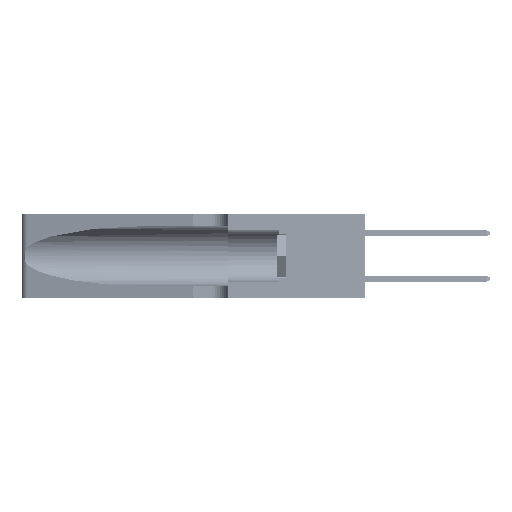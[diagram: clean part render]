
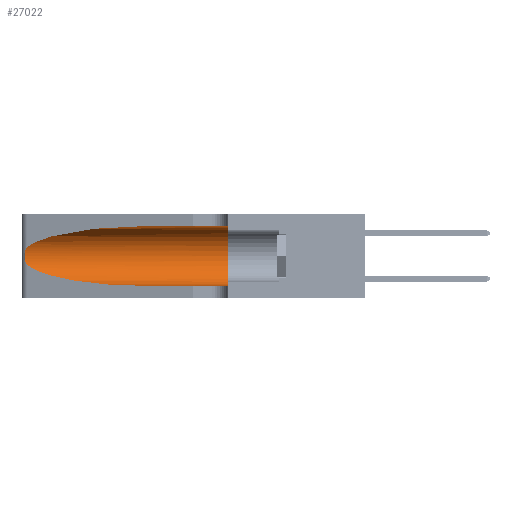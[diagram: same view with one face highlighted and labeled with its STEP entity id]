
A CAD part, left-side view. The second image highlights one B-rep face of the part: STEP entity #27022.
In plain terms, the highlighted cylindrical face has radius 3.308 mm (diameter 6.617 mm), a partial arc.
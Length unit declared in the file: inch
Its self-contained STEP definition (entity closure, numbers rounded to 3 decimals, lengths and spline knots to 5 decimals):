
#78 =( BOUNDED_CURVE ( )  B_SPLINE_CURVE ( 3, ( #13116, #714, #21134, #17236 ),
 .UNSPECIFIED., .F., .F. ) 
 B_SPLINE_CURVE_WITH_KNOTS ( ( 4, 4 ),
 ( 1.5708, 2.84003 ),
 .UNSPECIFIED. ) 
 CURVE ( )  GEOMETRIC_REPRESENTATION_ITEM ( )  RATIONAL_B_SPLINE_CURVE ( ( 1., 0.87, 0.87, 1. ) ) 
 REPRESENTATION_ITEM ( '' )  );
#714 = CARTESIAN_POINT ( 'NONE',  ( 0.18966, 0.96281, 0.31525 ) ) ;
#1242 = CARTESIAN_POINT ( 'NONE',  ( 0.25555, 1.22994, 0.2215 ) ) ;
#1420 = CARTESIAN_POINT ( 'NONE',  ( 0.25639, 1.23184, 0.21858 ) ) ;
#1897 = VECTOR ( 'NONE', #19409, 39.37008 ) ;
#2403 = VERTEX_POINT ( 'NONE', #41896 ) ;
#2942 = CARTESIAN_POINT ( 'NONE',  ( 0.1305, 1.61858, 0.31525 ) ) ;
#3427 = CIRCLE ( 'NONE', #12672, 0.13025 ) ;
#5554 = CARTESIAN_POINT ( 'NONE',  ( 0.25854, 1.2359, 0.20912 ) ) ;
#7035 = EDGE_LOOP ( 'NONE', ( #36587, #8484, #19408, #42284, #11086, #46083 ) ) ;
#7276 = CARTESIAN_POINT ( 'NONE',  ( 0.1305, 1.61858, 0.185 ) ) ;
#7532 = EDGE_CURVE ( 'NONE', #51830, #2403, #12821, .T. ) ;
#7982 =( BOUNDED_CURVE ( )  B_SPLINE_CURVE ( 3, ( #22563, #26666, #10369, #14528 ),
 .UNSPECIFIED., .F., .F. ) 
 B_SPLINE_CURVE_WITH_KNOTS ( ( 4, 4 ),
 ( 3.44316, 4.71239 ),
 .UNSPECIFIED. ) 
 CURVE ( )  GEOMETRIC_REPRESENTATION_ITEM ( )  RATIONAL_B_SPLINE_CURVE ( ( 1., 0.87, 0.87, 1. ) ) 
 REPRESENTATION_ITEM ( '' )  );
#8484 = ORIENTED_EDGE ( 'NONE', *, *, #44772, .T. ) ;
#9698 = CARTESIAN_POINT ( 'NONE',  ( 0.26075, 1.23896, 0.19203 ) ) ;
#9710 = CARTESIAN_POINT ( 'NONE',  ( 0.1305, 0.35, 0.185 ) ) ;
#10369 = CARTESIAN_POINT ( 'NONE',  ( 0.18966, 0.96281, 0.05475 ) ) ;
#10639 = CARTESIAN_POINT ( 'NONE',  ( 0.1305, 0.72297, 0.05475 ) ) ;
#11086 = ORIENTED_EDGE ( 'NONE', *, *, #27565, .F. ) ;
#12672 = AXIS2_PLACEMENT_3D ( 'NONE', #9710, #38253, #13833 ) ;
#12821 = LINE ( 'NONE', #2942, #1897 ) ;
#13116 = CARTESIAN_POINT ( 'NONE',  ( 0.1305, 0.72297, 0.31525 ) ) ;
#13673 = VERTEX_POINT ( 'NONE', #22888 ) ;
#13825 = CARTESIAN_POINT ( 'NONE',  ( 0.26017, 1.23833, 0.17102 ) ) ;
#13833 = DIRECTION ( 'NONE',  ( 0., 0., 1. ) ) ;
#14528 = CARTESIAN_POINT ( 'NONE',  ( 0.1305, 0.72297, 0.05475 ) ) ;
#17236 = CARTESIAN_POINT ( 'NONE',  ( 0.25487, 1.22718, 0.22369 ) ) ;
#17929 = CARTESIAN_POINT ( 'NONE',  ( 0.25789, 1.23486, 0.15765 ) ) ;
#19408 = ORIENTED_EDGE ( 'NONE', *, *, #19874, .T. ) ;
#19409 = DIRECTION ( 'NONE',  ( 0., -1., 0. ) ) ;
#19638 = EDGE_CURVE ( 'NONE', #51830, #47358, #78, .T. ) ;
#19874 = EDGE_CURVE ( 'NONE', #41516, #33897, #7982, .T. ) ;
#21134 = CARTESIAN_POINT ( 'NONE',  ( 0.2373, 1.15595, 0.28018 ) ) ;
#22030 = CARTESIAN_POINT ( 'NONE',  ( 0.25555, 1.22993, 0.14849 ) ) ;
#22563 = CARTESIAN_POINT ( 'NONE',  ( 0.25487, 1.22718, 0.14631 ) ) ;
#22888 = CARTESIAN_POINT ( 'NONE',  ( 0.1305, 0.35, 0.05475 ) ) ;
#22984 = CARTESIAN_POINT ( 'NONE',  ( 0.25487, 1.22718, 0.22369 ) ) ;
#26666 = CARTESIAN_POINT ( 'NONE',  ( 0.2373, 1.15595, 0.08982 ) ) ;
#27022 = ADVANCED_FACE ( 'NONE', ( #41116 ), #29119, .F. ) ;
#27441 = B_SPLINE_CURVE_WITH_KNOTS ( 'NONE', 3,
 ( #42065, #1242, #1420, #30077, #5554, #34178, #9698, #38243, #13825, #42237, #17929, #46283, #22030, #50346 ),
 .UNSPECIFIED., .F., .F.,
 ( 4, 2, 2, 2, 2, 2, 4 ),
 ( 0., 0.00027, 0.00053, 0.00107, 0.0016, 0.00187, 0.00214 ),
 .UNSPECIFIED. ) ;
#27565 = EDGE_CURVE ( 'NONE', #2403, #13673, #3427, .T. ) ;
#29119 = CYLINDRICAL_SURFACE ( 'NONE', #41955, 0.13025 ) ;
#30026 = EDGE_CURVE ( 'NONE', #33897, #13673, #30914, .T. ) ;
#30077 = CARTESIAN_POINT ( 'NONE',  ( 0.25787, 1.23484, 0.2124 ) ) ;
#30914 = LINE ( 'NONE', #37338, #40415 ) ;
#31779 = DIRECTION ( 'NONE',  ( 0., 0., -1. ) ) ;
#33897 = VERTEX_POINT ( 'NONE', #10639 ) ;
#34178 = CARTESIAN_POINT ( 'NONE',  ( 0.26018, 1.23835, 0.19895 ) ) ;
#36587 = ORIENTED_EDGE ( 'NONE', *, *, #19638, .T. ) ;
#37206 = CARTESIAN_POINT ( 'NONE',  ( 0.25487, 1.22718, 0.14631 ) ) ;
#37338 = CARTESIAN_POINT ( 'NONE',  ( 0.1305, 1.61858, 0.05475 ) ) ;
#38243 = CARTESIAN_POINT ( 'NONE',  ( 0.26075, 1.23896, 0.178 ) ) ;
#38253 = DIRECTION ( 'NONE',  ( 0., 1., 0. ) ) ;
#38976 = CARTESIAN_POINT ( 'NONE',  ( 0.1305, 0.72297, 0.31525 ) ) ;
#39923 = DIRECTION ( 'NONE',  ( 0., -1., 0. ) ) ;
#40415 = VECTOR ( 'NONE', #49440, 39.37008 ) ;
#41116 = FACE_OUTER_BOUND ( 'NONE', #7035, .T. ) ;
#41516 = VERTEX_POINT ( 'NONE', #37206 ) ;
#41896 = CARTESIAN_POINT ( 'NONE',  ( 0.1305, 0.35, 0.31525 ) ) ;
#41955 = AXIS2_PLACEMENT_3D ( 'NONE', #7276, #39923, #31779 ) ;
#42065 = CARTESIAN_POINT ( 'NONE',  ( 0.25487, 1.22718, 0.22369 ) ) ;
#42237 = CARTESIAN_POINT ( 'NONE',  ( 0.25856, 1.23593, 0.16098 ) ) ;
#42284 = ORIENTED_EDGE ( 'NONE', *, *, #30026, .T. ) ;
#44772 = EDGE_CURVE ( 'NONE', #47358, #41516, #27441, .T. ) ;
#46083 = ORIENTED_EDGE ( 'NONE', *, *, #7532, .F. ) ;
#46283 = CARTESIAN_POINT ( 'NONE',  ( 0.25639, 1.23186, 0.15144 ) ) ;
#47358 = VERTEX_POINT ( 'NONE', #22984 ) ;
#49440 = DIRECTION ( 'NONE',  ( 0., -1., 0. ) ) ;
#50346 = CARTESIAN_POINT ( 'NONE',  ( 0.25487, 1.22718, 0.14631 ) ) ;
#51830 = VERTEX_POINT ( 'NONE', #38976 ) ;
